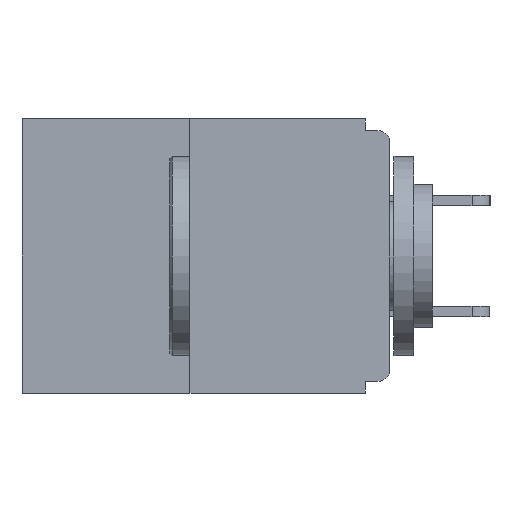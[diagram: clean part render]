
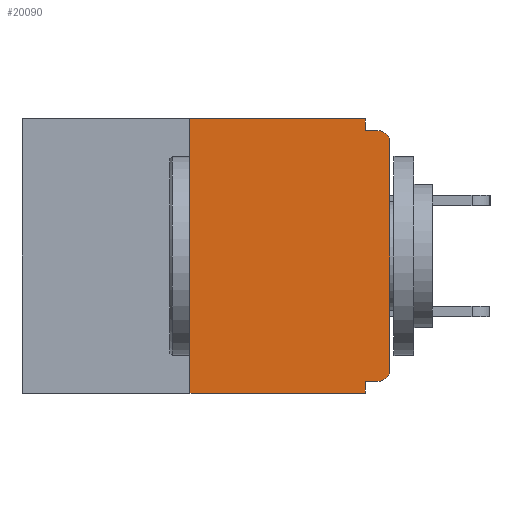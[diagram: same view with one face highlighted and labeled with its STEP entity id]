
A CAD part, left-side view. The second image highlights one B-rep face of the part: STEP entity #20090.
In plain terms, the highlighted planar face has unit normal (-1, 0, 0).
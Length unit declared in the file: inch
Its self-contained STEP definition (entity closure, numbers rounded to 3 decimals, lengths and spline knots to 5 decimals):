
#65 = CARTESIAN_POINT ( 'NONE',  ( 0., 0.25, 0. ) ) ;
#473 = LINE ( 'NONE', #65, #13754 ) ;
#545 = CARTESIAN_POINT ( 'NONE',  ( 0., 0., -0.313 ) ) ;
#717 = CARTESIAN_POINT ( 'NONE',  ( 0., 0.031, -0.328 ) ) ;
#888 = DIRECTION ( 'NONE',  ( -1., 0., 0. ) ) ;
#948 = EDGE_CURVE ( 'NONE', #14567, #4084, #12971, .T. ) ;
#1117 = DIRECTION ( 'NONE',  ( 0., 0., 1. ) ) ;
#1437 = LINE ( 'NONE', #15283, #17923 ) ;
#1881 = EDGE_CURVE ( 'NONE', #13871, #14567, #473, .T. ) ;
#1901 = AXIS2_PLACEMENT_3D ( 'NONE', #3575, #15662, #5302 ) ;
#2038 = ORIENTED_EDGE ( 'NONE', *, *, #12427, .T. ) ;
#2206 = CARTESIAN_POINT ( 'NONE',  ( 0., 0.015, -0.03 ) ) ;
#2214 = VECTOR ( 'NONE', #21950, 39.37008 ) ;
#2294 = LINE ( 'NONE', #6563, #11530 ) ;
#2672 = CARTESIAN_POINT ( 'NONE',  ( 0., 0.031, -0.015 ) ) ;
#3550 = CARTESIAN_POINT ( 'NONE',  ( 0., 0.25, -0.343 ) ) ;
#3575 = CARTESIAN_POINT ( 'NONE',  ( 0., 0.46, 0. ) ) ;
#3801 = VECTOR ( 'NONE', #21301, 39.37008 ) ;
#4084 = VERTEX_POINT ( 'NONE', #5503 ) ;
#4610 = ORIENTED_EDGE ( 'NONE', *, *, #1881, .F. ) ;
#5302 = DIRECTION ( 'NONE',  ( 0., 0., -1. ) ) ;
#5413 = CARTESIAN_POINT ( 'NONE',  ( 0., 0., -0.015 ) ) ;
#5503 = CARTESIAN_POINT ( 'NONE',  ( 0., 0.031, 0. ) ) ;
#6368 = AXIS2_PLACEMENT_3D ( 'NONE', #2206, #888, #11528 ) ;
#6563 = CARTESIAN_POINT ( 'NONE',  ( 0., 0., -0.328 ) ) ;
#6815 = LINE ( 'NONE', #15017, #2214 ) ;
#7248 = EDGE_CURVE ( 'NONE', #21128, #12498, #2294, .T. ) ;
#7692 = VECTOR ( 'NONE', #1117, 39.37008 ) ;
#7946 = VERTEX_POINT ( 'NONE', #10016 ) ;
#8263 = LINE ( 'NONE', #20063, #7692 ) ;
#8486 = ORIENTED_EDGE ( 'NONE', *, *, #7248, .F. ) ;
#9017 = ORIENTED_EDGE ( 'NONE', *, *, #9810, .F. ) ;
#9174 = DIRECTION ( 'NONE',  ( 0., -1., 0. ) ) ;
#9213 = DIRECTION ( 'NONE',  ( -1., 0., 0. ) ) ;
#9328 = VERTEX_POINT ( 'NONE', #545 ) ;
#9564 = DIRECTION ( 'NONE',  ( 0., 0., -1. ) ) ;
#9810 = EDGE_CURVE ( 'NONE', #10449, #20396, #15936, .T. ) ;
#10016 = CARTESIAN_POINT ( 'NONE',  ( 0., 0.031, -0.343 ) ) ;
#10336 = CARTESIAN_POINT ( 'NONE',  ( 0., 0., -0.03 ) ) ;
#10449 = VERTEX_POINT ( 'NONE', #2672 ) ;
#11277 = CARTESIAN_POINT ( 'NONE',  ( 0., 0.015, -0.328 ) ) ;
#11317 = CARTESIAN_POINT ( 'NONE',  ( 0., 0.031, 0. ) ) ;
#11355 = VECTOR ( 'NONE', #9174, 39.37008 ) ;
#11528 = DIRECTION ( 'NONE',  ( 0., 0., -1. ) ) ;
#11530 = VECTOR ( 'NONE', #16863, 39.37008 ) ;
#12427 = EDGE_CURVE ( 'NONE', #21128, #9328, #21493, .T. ) ;
#12482 = DIRECTION ( 'NONE',  ( 0., 0., -1. ) ) ;
#12498 = VERTEX_POINT ( 'NONE', #717 ) ;
#12511 = ORIENTED_EDGE ( 'NONE', *, *, #21949, .F. ) ;
#12971 = LINE ( 'NONE', #18117, #3801 ) ;
#13164 = LINE ( 'NONE', #11317, #21811 ) ;
#13703 = ORIENTED_EDGE ( 'NONE', *, *, #18510, .T. ) ;
#13754 = VECTOR ( 'NONE', #18998, 39.37008 ) ;
#13845 = ORIENTED_EDGE ( 'NONE', *, *, #948, .F. ) ;
#13849 = PLANE ( 'NONE',  #1901 ) ;
#13871 = VERTEX_POINT ( 'NONE', #3550 ) ;
#13873 = AXIS2_PLACEMENT_3D ( 'NONE', #19589, #9213, #12482 ) ;
#14567 = VERTEX_POINT ( 'NONE', #18293 ) ;
#14709 = EDGE_CURVE ( 'NONE', #13871, #7946, #1437, .T. ) ;
#15017 = CARTESIAN_POINT ( 'NONE',  ( 0., 0.031, -0.343 ) ) ;
#15217 = ORIENTED_EDGE ( 'NONE', *, *, #17812, .F. ) ;
#15272 = VERTEX_POINT ( 'NONE', #10336 ) ;
#15283 = CARTESIAN_POINT ( 'NONE',  ( 0., 0.46, -0.343 ) ) ;
#15605 = CIRCLE ( 'NONE', #6368, 0.015 ) ;
#15662 = DIRECTION ( 'NONE',  ( 1., 0., 0. ) ) ;
#15936 = LINE ( 'NONE', #5413, #11355 ) ;
#16285 = EDGE_LOOP ( 'NONE', ( #13845, #4610, #19420, #12511, #8486, #2038, #13703, #17937, #9017, #15217 ) ) ;
#16863 = DIRECTION ( 'NONE',  ( 0., 1., 0. ) ) ;
#17650 = EDGE_CURVE ( 'NONE', #15272, #20396, #15605, .T. ) ;
#17812 = EDGE_CURVE ( 'NONE', #4084, #10449, #13164, .T. ) ;
#17923 = VECTOR ( 'NONE', #18591, 39.37008 ) ;
#17937 = ORIENTED_EDGE ( 'NONE', *, *, #17650, .T. ) ;
#18117 = CARTESIAN_POINT ( 'NONE',  ( 0., 0.46, 0. ) ) ;
#18293 = CARTESIAN_POINT ( 'NONE',  ( 0., 0.25, 0. ) ) ;
#18510 = EDGE_CURVE ( 'NONE', #9328, #15272, #8263, .T. ) ;
#18591 = DIRECTION ( 'NONE',  ( 0., -1., 0. ) ) ;
#18998 = DIRECTION ( 'NONE',  ( 0., 0., 1. ) ) ;
#19420 = ORIENTED_EDGE ( 'NONE', *, *, #14709, .T. ) ;
#19589 = CARTESIAN_POINT ( 'NONE',  ( 0., 0.015, -0.313 ) ) ;
#20063 = CARTESIAN_POINT ( 'NONE',  ( 0., 0., 0. ) ) ;
#20090 = ADVANCED_FACE ( 'NONE', ( #22247 ), #13849, .F. ) ;
#20396 = VERTEX_POINT ( 'NONE', #21620 ) ;
#21128 = VERTEX_POINT ( 'NONE', #11277 ) ;
#21301 = DIRECTION ( 'NONE',  ( 0., -1., 0. ) ) ;
#21493 = CIRCLE ( 'NONE', #13873, 0.015 ) ;
#21620 = CARTESIAN_POINT ( 'NONE',  ( 0., 0.015, -0.015 ) ) ;
#21811 = VECTOR ( 'NONE', #9564, 39.37008 ) ;
#21949 = EDGE_CURVE ( 'NONE', #12498, #7946, #6815, .T. ) ;
#21950 = DIRECTION ( 'NONE',  ( 0., 0., -1. ) ) ;
#22247 = FACE_OUTER_BOUND ( 'NONE', #16285, .T. ) ;
